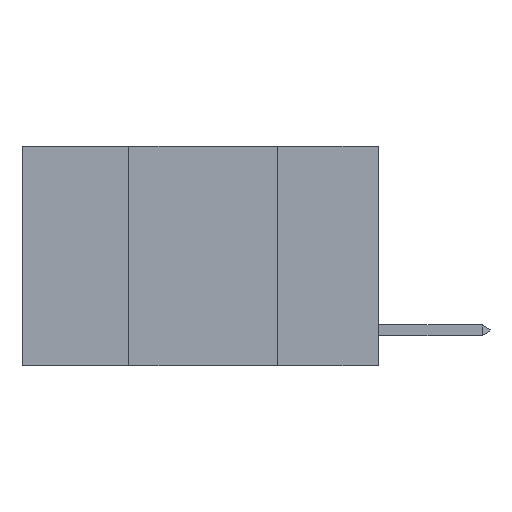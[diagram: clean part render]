
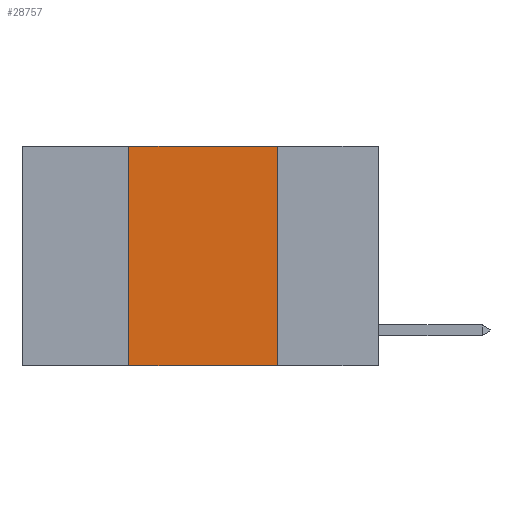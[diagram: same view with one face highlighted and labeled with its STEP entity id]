
A CAD part, left-side view. The second image highlights one B-rep face of the part: STEP entity #28757.
In plain terms, the highlighted planar face has unit normal (-1, 0, 0).
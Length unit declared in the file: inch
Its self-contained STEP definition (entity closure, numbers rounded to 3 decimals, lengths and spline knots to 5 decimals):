
#212 = LINE ( 'NONE', #16581, #16906 ) ;
#606 = DIRECTION ( 'NONE',  ( 0., 0., -1. ) ) ;
#950 = VECTOR ( 'NONE', #16210, 39.37008 ) ;
#2590 = VERTEX_POINT ( 'NONE', #27500 ) ;
#2880 = ORIENTED_EDGE ( 'NONE', *, *, #18668, .F. ) ;
#3414 = EDGE_CURVE ( 'NONE', #2590, #9931, #11450, .T. ) ;
#4585 = DIRECTION ( 'NONE',  ( 0., -1., 0. ) ) ;
#5471 = PLANE ( 'NONE',  #12723 ) ;
#5678 = EDGE_LOOP ( 'NONE', ( #25253, #2880, #29381, #13768 ) ) ;
#6994 = VERTEX_POINT ( 'NONE', #21672 ) ;
#7142 = CARTESIAN_POINT ( 'NONE',  ( 0., 0.6, 0. ) ) ;
#9114 = EDGE_CURVE ( 'NONE', #2590, #6994, #212, .T. ) ;
#9366 = CARTESIAN_POINT ( 'NONE',  ( 0., 0.6, -0.37 ) ) ;
#9632 = CARTESIAN_POINT ( 'NONE',  ( 0., 0.17, 0. ) ) ;
#9931 = VERTEX_POINT ( 'NONE', #11112 ) ;
#10090 = VECTOR ( 'NONE', #18413, 39.37008 ) ;
#11112 = CARTESIAN_POINT ( 'NONE',  ( 0., 0.17, -0.37 ) ) ;
#11450 = LINE ( 'NONE', #9366, #950 ) ;
#11631 = DIRECTION ( 'NONE',  ( 1., 0., 0. ) ) ;
#11729 = VECTOR ( 'NONE', #4585, 39.37008 ) ;
#12723 = AXIS2_PLACEMENT_3D ( 'NONE', #7142, #11631, #606 ) ;
#13768 = ORIENTED_EDGE ( 'NONE', *, *, #3414, .T. ) ;
#13842 = CARTESIAN_POINT ( 'NONE',  ( 0., 0.6, 0. ) ) ;
#14040 = EDGE_CURVE ( 'NONE', #21812, #9931, #24277, .T. ) ;
#16210 = DIRECTION ( 'NONE',  ( 0., -1., 0. ) ) ;
#16581 = CARTESIAN_POINT ( 'NONE',  ( 0., 0.42, 0. ) ) ;
#16906 = VECTOR ( 'NONE', #27355, 39.37008 ) ;
#18413 = DIRECTION ( 'NONE',  ( 0., 0., -1. ) ) ;
#18492 = FACE_OUTER_BOUND ( 'NONE', #5678, .T. ) ;
#18668 = EDGE_CURVE ( 'NONE', #6994, #21812, #29362, .T. ) ;
#20643 = CARTESIAN_POINT ( 'NONE',  ( 0., 0.17, 0. ) ) ;
#21672 = CARTESIAN_POINT ( 'NONE',  ( 0., 0.42, 0. ) ) ;
#21812 = VERTEX_POINT ( 'NONE', #9632 ) ;
#24277 = LINE ( 'NONE', #20643, #10090 ) ;
#25253 = ORIENTED_EDGE ( 'NONE', *, *, #14040, .F. ) ;
#27355 = DIRECTION ( 'NONE',  ( 0., 0., 1. ) ) ;
#27500 = CARTESIAN_POINT ( 'NONE',  ( 0., 0.42, -0.37 ) ) ;
#28757 = ADVANCED_FACE ( 'NONE', ( #18492 ), #5471, .F. ) ;
#29362 = LINE ( 'NONE', #13842, #11729 ) ;
#29381 = ORIENTED_EDGE ( 'NONE', *, *, #9114, .F. ) ;
